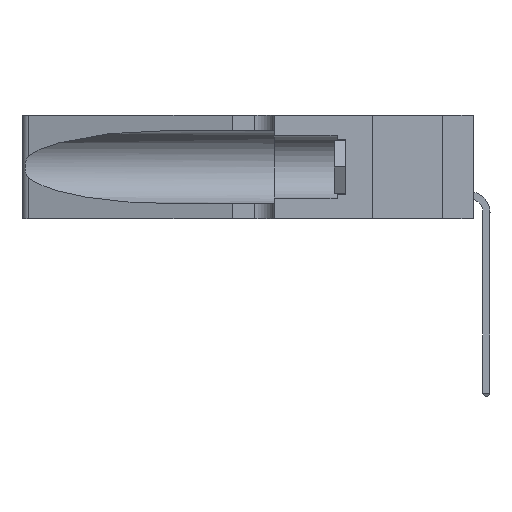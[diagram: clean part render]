
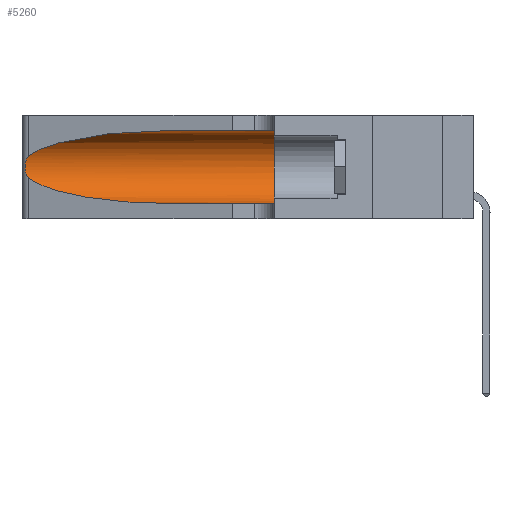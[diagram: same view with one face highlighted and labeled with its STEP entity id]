
A CAD part, left-side view. The second image highlights one B-rep face of the part: STEP entity #5260.
In plain terms, the highlighted cylindrical face has radius 3.308 mm (diameter 6.617 mm), a partial arc.
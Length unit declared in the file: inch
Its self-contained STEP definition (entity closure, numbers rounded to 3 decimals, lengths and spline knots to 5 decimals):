
#318 = B_SPLINE_CURVE_WITH_KNOTS ( 'NONE', 3,
 ( #12208, #42071, #38345, #25089, #2546, #2397, #15809, #35426, #18710, #8743, #2692, #15373, #12489, #22243 ),
 .UNSPECIFIED., .F., .F.,
 ( 4, 2, 2, 2, 2, 2, 4 ),
 ( 0., 0.00027, 0.00053, 0.00107, 0.0016, 0.00187, 0.00214 ),
 .UNSPECIFIED. ) ;
#571 = VERTEX_POINT ( 'NONE', #38412 ) ;
#720 = CARTESIAN_POINT ( 'NONE',  ( 0.2373, 1.15595, 0.28018 ) ) ;
#2397 = CARTESIAN_POINT ( 'NONE',  ( 0.26018, 1.23835, 0.19895 ) ) ;
#2445 = CARTESIAN_POINT ( 'NONE',  ( 0.25487, 1.22718, 0.22369 ) ) ;
#2546 = CARTESIAN_POINT ( 'NONE',  ( 0.25854, 1.2359, 0.20912 ) ) ;
#2692 = CARTESIAN_POINT ( 'NONE',  ( 0.25789, 1.23486, 0.15765 ) ) ;
#4017 = VERTEX_POINT ( 'NONE', #39730 ) ;
#5260 = ADVANCED_FACE ( 'NONE', ( #20508 ), #36321, .F. ) ;
#5502 = DIRECTION ( 'NONE',  ( 0., 0., 1. ) ) ;
#7027 = EDGE_LOOP ( 'NONE', ( #26665, #42122, #39268, #40498, #20328, #9710 ) ) ;
#7877 = CARTESIAN_POINT ( 'NONE',  ( 0.1305, 0.35, 0.05475 ) ) ;
#8355 = VERTEX_POINT ( 'NONE', #7877 ) ;
#8743 = CARTESIAN_POINT ( 'NONE',  ( 0.25856, 1.23593, 0.16098 ) ) ;
#9710 = ORIENTED_EDGE ( 'NONE', *, *, #30647, .F. ) ;
#10061 = VERTEX_POINT ( 'NONE', #23812 ) ;
#11131 = AXIS2_PLACEMENT_3D ( 'NONE', #38436, #25174, #5502 ) ;
#11142 = CARTESIAN_POINT ( 'NONE',  ( 0.1305, 1.61858, 0.31525 ) ) ;
#12208 = CARTESIAN_POINT ( 'NONE',  ( 0.25487, 1.22718, 0.22369 ) ) ;
#12245 = EDGE_CURVE ( 'NONE', #571, #8355, #18268, .T. ) ;
#12489 = CARTESIAN_POINT ( 'NONE',  ( 0.25555, 1.22993, 0.14849 ) ) ;
#12492 =( BOUNDED_CURVE ( )  B_SPLINE_CURVE ( 3, ( #36255, #12758, #17061, #39875 ),
 .UNSPECIFIED., .F., .F. ) 
 B_SPLINE_CURVE_WITH_KNOTS ( ( 4, 4 ),
 ( 3.44316, 4.71239 ),
 .UNSPECIFIED. ) 
 CURVE ( )  GEOMETRIC_REPRESENTATION_ITEM ( )  RATIONAL_B_SPLINE_CURVE ( ( 1., 0.87, 0.87, 1. ) ) 
 REPRESENTATION_ITEM ( '' )  );
#12758 = CARTESIAN_POINT ( 'NONE',  ( 0.2373, 1.15595, 0.08982 ) ) ;
#15373 = CARTESIAN_POINT ( 'NONE',  ( 0.25639, 1.23186, 0.15144 ) ) ;
#15809 = CARTESIAN_POINT ( 'NONE',  ( 0.26075, 1.23896, 0.19203 ) ) ;
#16756 = CARTESIAN_POINT ( 'NONE',  ( 0.18966, 0.96281, 0.31525 ) ) ;
#17061 = CARTESIAN_POINT ( 'NONE',  ( 0.18966, 0.96281, 0.05475 ) ) ;
#18268 = CIRCLE ( 'NONE', #11131, 0.13025 ) ;
#18314 =( BOUNDED_CURVE ( )  B_SPLINE_CURVE ( 3, ( #42609, #16756, #720, #27301 ),
 .UNSPECIFIED., .F., .T. ) 
 B_SPLINE_CURVE_WITH_KNOTS ( ( 4, 4 ),
 ( 1.5708, 2.84003 ),
 .UNSPECIFIED. ) 
 CURVE ( )  GEOMETRIC_REPRESENTATION_ITEM ( )  RATIONAL_B_SPLINE_CURVE ( ( 1., 0.87, 0.87, 1. ) ) 
 REPRESENTATION_ITEM ( '' )  );
#18710 = CARTESIAN_POINT ( 'NONE',  ( 0.26017, 1.23833, 0.17102 ) ) ;
#20328 = ORIENTED_EDGE ( 'NONE', *, *, #12245, .F. ) ;
#20508 = FACE_OUTER_BOUND ( 'NONE', #7027, .T. ) ;
#20661 = EDGE_CURVE ( 'NONE', #10061, #37292, #12492, .T. ) ;
#21236 = DIRECTION ( 'NONE',  ( 0., -1., 0. ) ) ;
#21352 = LINE ( 'NONE', #34800, #25965 ) ;
#22243 = CARTESIAN_POINT ( 'NONE',  ( 0.25487, 1.22718, 0.14631 ) ) ;
#23812 = CARTESIAN_POINT ( 'NONE',  ( 0.25487, 1.22718, 0.14631 ) ) ;
#24945 = CARTESIAN_POINT ( 'NONE',  ( 0.1305, 1.61858, 0.185 ) ) ;
#25089 = CARTESIAN_POINT ( 'NONE',  ( 0.25787, 1.23484, 0.2124 ) ) ;
#25174 = DIRECTION ( 'NONE',  ( 0., 1., 0. ) ) ;
#25965 = VECTOR ( 'NONE', #31621, 39.37008 ) ;
#26665 = ORIENTED_EDGE ( 'NONE', *, *, #27599, .T. ) ;
#27301 = CARTESIAN_POINT ( 'NONE',  ( 0.25487, 1.22718, 0.22369 ) ) ;
#27599 = EDGE_CURVE ( 'NONE', #4017, #27951, #18314, .T. ) ;
#27809 = DIRECTION ( 'NONE',  ( 0., 0., -1. ) ) ;
#27951 = VERTEX_POINT ( 'NONE', #2445 ) ;
#30167 = EDGE_CURVE ( 'NONE', #27951, #10061, #318, .T. ) ;
#30647 = EDGE_CURVE ( 'NONE', #4017, #571, #41042, .T. ) ;
#31060 = CARTESIAN_POINT ( 'NONE',  ( 0.1305, 0.72297, 0.05475 ) ) ;
#31621 = DIRECTION ( 'NONE',  ( 0., -1., 0. ) ) ;
#34800 = CARTESIAN_POINT ( 'NONE',  ( 0.1305, 1.61858, 0.05475 ) ) ;
#35426 = CARTESIAN_POINT ( 'NONE',  ( 0.26075, 1.23896, 0.178 ) ) ;
#36255 = CARTESIAN_POINT ( 'NONE',  ( 0.25487, 1.22718, 0.14631 ) ) ;
#36321 = CYLINDRICAL_SURFACE ( 'NONE', #36799, 0.13025 ) ;
#36799 = AXIS2_PLACEMENT_3D ( 'NONE', #24945, #21236, #27809 ) ;
#37292 = VERTEX_POINT ( 'NONE', #31060 ) ;
#38345 = CARTESIAN_POINT ( 'NONE',  ( 0.25639, 1.23184, 0.21858 ) ) ;
#38412 = CARTESIAN_POINT ( 'NONE',  ( 0.1305, 0.35, 0.31525 ) ) ;
#38436 = CARTESIAN_POINT ( 'NONE',  ( 0.1305, 0.35, 0.185 ) ) ;
#38972 = VECTOR ( 'NONE', #40893, 39.37008 ) ;
#39268 = ORIENTED_EDGE ( 'NONE', *, *, #20661, .T. ) ;
#39730 = CARTESIAN_POINT ( 'NONE',  ( 0.1305, 0.72297, 0.31525 ) ) ;
#39875 = CARTESIAN_POINT ( 'NONE',  ( 0.1305, 0.72297, 0.05475 ) ) ;
#40498 = ORIENTED_EDGE ( 'NONE', *, *, #41309, .T. ) ;
#40893 = DIRECTION ( 'NONE',  ( 0., -1., 0. ) ) ;
#41042 = LINE ( 'NONE', #11142, #38972 ) ;
#41309 = EDGE_CURVE ( 'NONE', #37292, #8355, #21352, .T. ) ;
#42071 = CARTESIAN_POINT ( 'NONE',  ( 0.25555, 1.22994, 0.2215 ) ) ;
#42122 = ORIENTED_EDGE ( 'NONE', *, *, #30167, .T. ) ;
#42609 = CARTESIAN_POINT ( 'NONE',  ( 0.1305, 0.72297, 0.31525 ) ) ;
